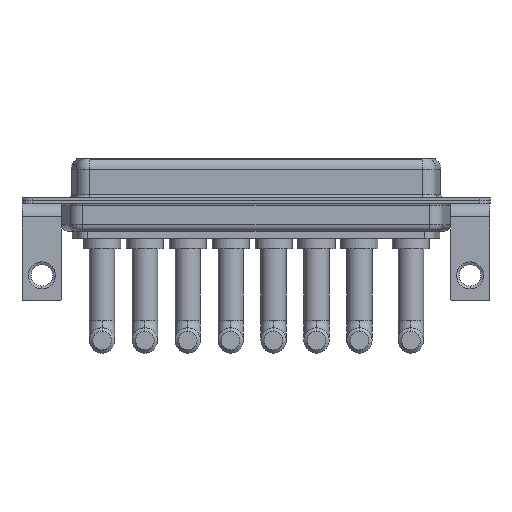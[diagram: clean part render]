
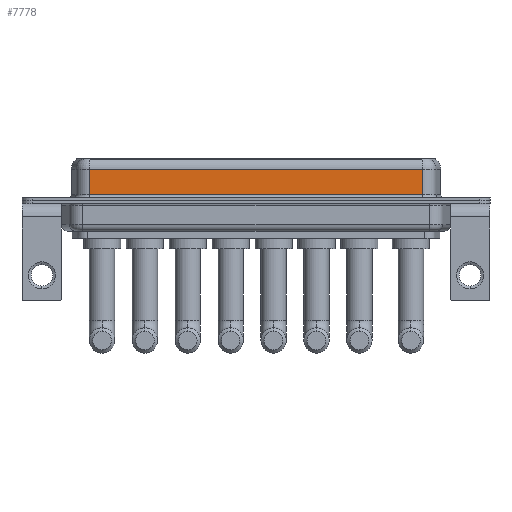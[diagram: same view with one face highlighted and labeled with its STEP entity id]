
A CAD part, front view. The second image highlights one B-rep face of the part: STEP entity #7778.
In plain terms, the highlighted planar face has unit normal (0, -1, 0).
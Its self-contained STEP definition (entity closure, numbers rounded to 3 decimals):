
#128 = ORIENTED_EDGE ( 'NONE', *, *, #4221, .T. ) ;
#336 = ORIENTED_EDGE ( 'NONE', *, *, #424, .F. ) ;
#398 = DIRECTION ( 'NONE',  ( -1., 0., 0. ) ) ;
#424 = EDGE_CURVE ( 'NONE', #9642, #4795, #830, .T. ) ;
#830 = LINE ( 'NONE', #13701, #13262 ) ;
#893 = CARTESIAN_POINT ( 'NONE',  ( 7.038, -3.95, 6.4 ) ) ;
#916 = VECTOR ( 'NONE', #5235, 1000. ) ;
#1501 = ORIENTED_EDGE ( 'NONE', *, *, #7388, .T. ) ;
#1513 = CARTESIAN_POINT ( 'NONE',  ( 7.038, -3.95, 0.9 ) ) ;
#2314 = CARTESIAN_POINT ( 'NONE',  ( 56.462, -3.95, 4.65 ) ) ;
#2570 = CARTESIAN_POINT ( 'NONE',  ( 56.462, -3.95, 0.9 ) ) ;
#3736 = DIRECTION ( 'NONE',  ( 0., 0., -1. ) ) ;
#3930 = FACE_OUTER_BOUND ( 'NONE', #10791, .T. ) ;
#4033 = VECTOR ( 'NONE', #398, 1000. ) ;
#4221 = EDGE_CURVE ( 'NONE', #9642, #7649, #12057, .T. ) ;
#4795 = VERTEX_POINT ( 'NONE', #2570 ) ;
#4998 = VERTEX_POINT ( 'NONE', #1513 ) ;
#5081 = CARTESIAN_POINT ( 'NONE',  ( 56.462, -3.95, 6.4 ) ) ;
#5235 = DIRECTION ( 'NONE',  ( 0., 0., -1. ) ) ;
#5999 = DIRECTION ( 'NONE',  ( 0., 1., 0. ) ) ;
#6276 = LINE ( 'NONE', #10678, #7860 ) ;
#6968 = CARTESIAN_POINT ( 'NONE',  ( 56.462, -3.95, 4.65 ) ) ;
#7388 = EDGE_CURVE ( 'NONE', #7649, #4998, #12759, .T. ) ;
#7649 = VERTEX_POINT ( 'NONE', #12324 ) ;
#7778 = ADVANCED_FACE ( 'NONE', ( #3930 ), #12595, .F. ) ;
#7860 = VECTOR ( 'NONE', #8621, 1000. ) ;
#8472 = AXIS2_PLACEMENT_3D ( 'NONE', #5081, #5999, #12457 ) ;
#8621 = DIRECTION ( 'NONE',  ( 1., 0., 0. ) ) ;
#9306 = EDGE_CURVE ( 'NONE', #4998, #4795, #6276, .T. ) ;
#9642 = VERTEX_POINT ( 'NONE', #6968 ) ;
#10678 = CARTESIAN_POINT ( 'NONE',  ( 56.462, -3.95, 0.9 ) ) ;
#10791 = EDGE_LOOP ( 'NONE', ( #336, #128, #1501, #12129 ) ) ;
#12057 = LINE ( 'NONE', #2314, #4033 ) ;
#12129 = ORIENTED_EDGE ( 'NONE', *, *, #9306, .T. ) ;
#12324 = CARTESIAN_POINT ( 'NONE',  ( 7.038, -3.95, 4.65 ) ) ;
#12457 = DIRECTION ( 'NONE',  ( 0., 0., 1. ) ) ;
#12595 = PLANE ( 'NONE',  #8472 ) ;
#12759 = LINE ( 'NONE', #893, #916 ) ;
#13262 = VECTOR ( 'NONE', #3736, 1000. ) ;
#13701 = CARTESIAN_POINT ( 'NONE',  ( 56.462, -3.95, 6.4 ) ) ;
